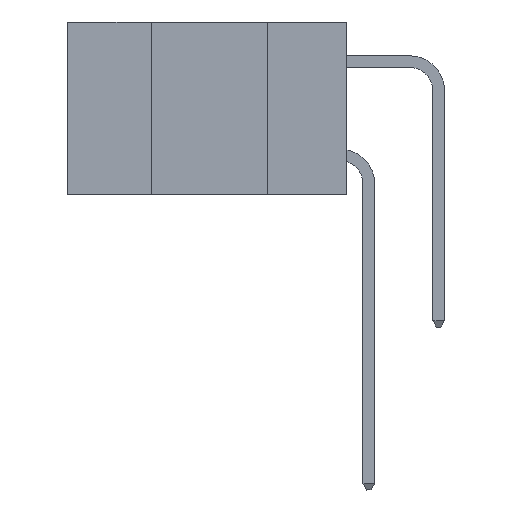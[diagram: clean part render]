
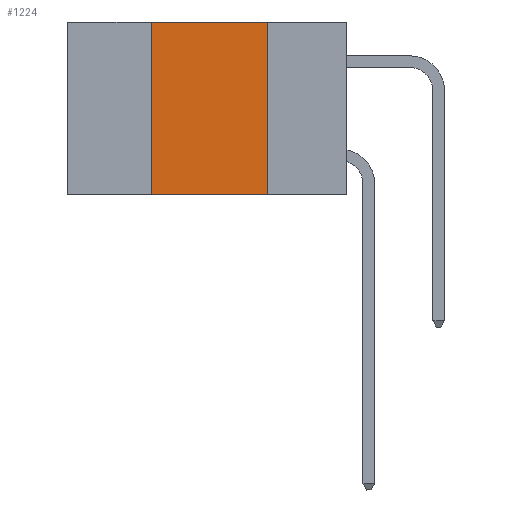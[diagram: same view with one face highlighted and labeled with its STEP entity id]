
A CAD part, left-side view. The second image highlights one B-rep face of the part: STEP entity #1224.
In plain terms, the highlighted planar face has unit normal (-1, 0, 0).
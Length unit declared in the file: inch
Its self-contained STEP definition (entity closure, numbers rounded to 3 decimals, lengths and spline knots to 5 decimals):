
#437 = DIRECTION ( 'NONE',  ( 0., 0., 1. ) ) ;
#1224 = ADVANCED_FACE ( 'NONE', ( #6710 ), #16941, .F. ) ;
#2323 = VERTEX_POINT ( 'NONE', #7975 ) ;
#3393 = EDGE_CURVE ( 'NONE', #18047, #2323, #22269, .T. ) ;
#3510 = ORIENTED_EDGE ( 'NONE', *, *, #23067, .F. ) ;
#4139 = VECTOR ( 'NONE', #15421, 39.37008 ) ;
#4575 = EDGE_CURVE ( 'NONE', #9324, #27174, #19620, .T. ) ;
#5553 = LINE ( 'NONE', #25101, #4139 ) ;
#6567 = VECTOR ( 'NONE', #11088, 39.37008 ) ;
#6710 = FACE_OUTER_BOUND ( 'NONE', #11501, .T. ) ;
#7011 = LINE ( 'NONE', #7156, #20155 ) ;
#7156 = CARTESIAN_POINT ( 'NONE',  ( 0., 0.42, 0. ) ) ;
#7975 = CARTESIAN_POINT ( 'NONE',  ( 0., 0.17, -0.37 ) ) ;
#9324 = VERTEX_POINT ( 'NONE', #23083 ) ;
#10032 = ORIENTED_EDGE ( 'NONE', *, *, #4575, .F. ) ;
#10289 = DIRECTION ( 'NONE',  ( 1., 0., 0. ) ) ;
#10868 = AXIS2_PLACEMENT_3D ( 'NONE', #21950, #10289, #20007 ) ;
#11088 = DIRECTION ( 'NONE',  ( 0., -1., 0. ) ) ;
#11501 = EDGE_LOOP ( 'NONE', ( #30119, #10032, #3510, #24587 ) ) ;
#11592 = CARTESIAN_POINT ( 'NONE',  ( 0., 0.17, 0. ) ) ;
#14480 = VECTOR ( 'NONE', #24344, 39.37008 ) ;
#15421 = DIRECTION ( 'NONE',  ( 0., 0., -1. ) ) ;
#16941 = PLANE ( 'NONE',  #10868 ) ;
#18047 = VERTEX_POINT ( 'NONE', #29568 ) ;
#18444 = CARTESIAN_POINT ( 'NONE',  ( 0., 0.6, -0.37 ) ) ;
#19620 = LINE ( 'NONE', #29479, #14480 ) ;
#20007 = DIRECTION ( 'NONE',  ( 0., 0., -1. ) ) ;
#20155 = VECTOR ( 'NONE', #437, 39.37008 ) ;
#21950 = CARTESIAN_POINT ( 'NONE',  ( 0., 0.6, 0. ) ) ;
#22269 = LINE ( 'NONE', #18444, #6567 ) ;
#22809 = EDGE_CURVE ( 'NONE', #27174, #2323, #5553, .T. ) ;
#23067 = EDGE_CURVE ( 'NONE', #18047, #9324, #7011, .T. ) ;
#23083 = CARTESIAN_POINT ( 'NONE',  ( 0., 0.42, 0. ) ) ;
#24344 = DIRECTION ( 'NONE',  ( 0., -1., 0. ) ) ;
#24587 = ORIENTED_EDGE ( 'NONE', *, *, #3393, .T. ) ;
#25101 = CARTESIAN_POINT ( 'NONE',  ( 0., 0.17, 0. ) ) ;
#27174 = VERTEX_POINT ( 'NONE', #11592 ) ;
#29479 = CARTESIAN_POINT ( 'NONE',  ( 0., 0.6, 0. ) ) ;
#29568 = CARTESIAN_POINT ( 'NONE',  ( 0., 0.42, -0.37 ) ) ;
#30119 = ORIENTED_EDGE ( 'NONE', *, *, #22809, .F. ) ;
